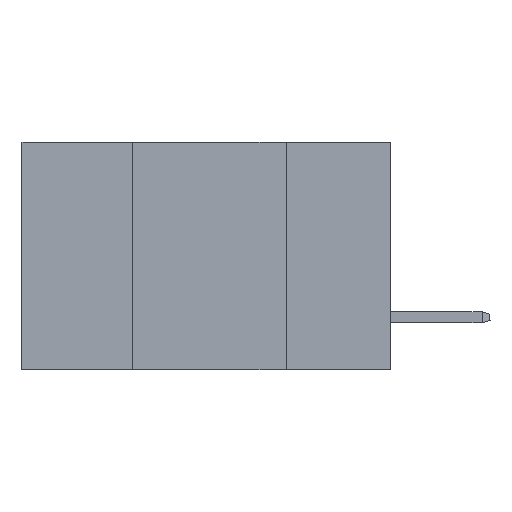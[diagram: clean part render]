
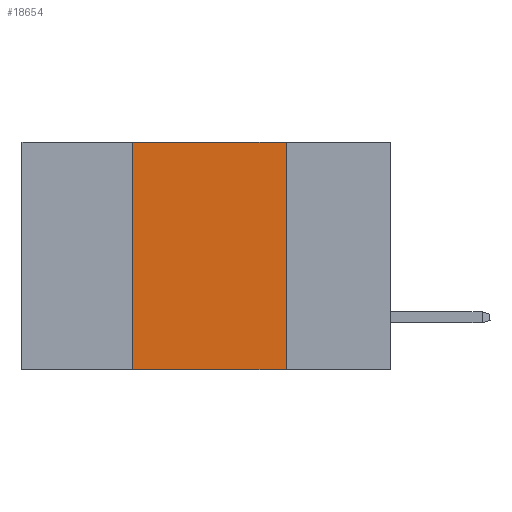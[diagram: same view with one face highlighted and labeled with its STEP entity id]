
A CAD part, left-side view. The second image highlights one B-rep face of the part: STEP entity #18654.
In plain terms, the highlighted planar face has unit normal (-1, 0, 0).
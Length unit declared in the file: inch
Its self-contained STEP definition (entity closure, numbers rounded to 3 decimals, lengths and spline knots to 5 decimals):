
#590 = CARTESIAN_POINT ( 'NONE',  ( 0., 0.6, -0.37 ) ) ;
#1768 = ORIENTED_EDGE ( 'NONE', *, *, #13358, .F. ) ;
#2211 = EDGE_LOOP ( 'NONE', ( #3001, #25609, #1768, #23313 ) ) ;
#2327 = LINE ( 'NONE', #5450, #22734 ) ;
#2385 = DIRECTION ( 'NONE',  ( 0., 0., 1. ) ) ;
#2694 = CARTESIAN_POINT ( 'NONE',  ( 0., 0.42, -0.37 ) ) ;
#3001 = ORIENTED_EDGE ( 'NONE', *, *, #7169, .F. ) ;
#3760 = FACE_OUTER_BOUND ( 'NONE', #2211, .T. ) ;
#5450 = CARTESIAN_POINT ( 'NONE',  ( 0., 0.17, 0. ) ) ;
#6146 = VECTOR ( 'NONE', #2385, 39.37008 ) ;
#7169 = EDGE_CURVE ( 'NONE', #20789, #8711, #2327, .T. ) ;
#7639 = VERTEX_POINT ( 'NONE', #10898 ) ;
#8434 = AXIS2_PLACEMENT_3D ( 'NONE', #15799, #19579, #23471 ) ;
#8521 = DIRECTION ( 'NONE',  ( 0., -1., 0. ) ) ;
#8711 = VERTEX_POINT ( 'NONE', #13544 ) ;
#9117 = EDGE_CURVE ( 'NONE', #22540, #8711, #15832, .T. ) ;
#10898 = CARTESIAN_POINT ( 'NONE',  ( 0., 0.42, 0. ) ) ;
#11774 = PLANE ( 'NONE',  #8434 ) ;
#12062 = LINE ( 'NONE', #21997, #6146 ) ;
#13358 = EDGE_CURVE ( 'NONE', #22540, #7639, #12062, .T. ) ;
#13544 = CARTESIAN_POINT ( 'NONE',  ( 0., 0.17, -0.37 ) ) ;
#14771 = DIRECTION ( 'NONE',  ( 0., -1., 0. ) ) ;
#15799 = CARTESIAN_POINT ( 'NONE',  ( 0., 0.6, 0. ) ) ;
#15832 = LINE ( 'NONE', #590, #19830 ) ;
#16801 = CARTESIAN_POINT ( 'NONE',  ( 0., 0.6, 0. ) ) ;
#17272 = DIRECTION ( 'NONE',  ( 0., 0., -1. ) ) ;
#17357 = VECTOR ( 'NONE', #14771, 39.37008 ) ;
#18654 = ADVANCED_FACE ( 'NONE', ( #3760 ), #11774, .F. ) ;
#18734 = CARTESIAN_POINT ( 'NONE',  ( 0., 0.17, 0. ) ) ;
#19086 = EDGE_CURVE ( 'NONE', #7639, #20789, #25363, .T. ) ;
#19579 = DIRECTION ( 'NONE',  ( 1., 0., 0. ) ) ;
#19830 = VECTOR ( 'NONE', #8521, 39.37008 ) ;
#20789 = VERTEX_POINT ( 'NONE', #18734 ) ;
#21997 = CARTESIAN_POINT ( 'NONE',  ( 0., 0.42, 0. ) ) ;
#22540 = VERTEX_POINT ( 'NONE', #2694 ) ;
#22734 = VECTOR ( 'NONE', #17272, 39.37008 ) ;
#23313 = ORIENTED_EDGE ( 'NONE', *, *, #9117, .T. ) ;
#23471 = DIRECTION ( 'NONE',  ( 0., 0., -1. ) ) ;
#25363 = LINE ( 'NONE', #16801, #17357 ) ;
#25609 = ORIENTED_EDGE ( 'NONE', *, *, #19086, .F. ) ;
